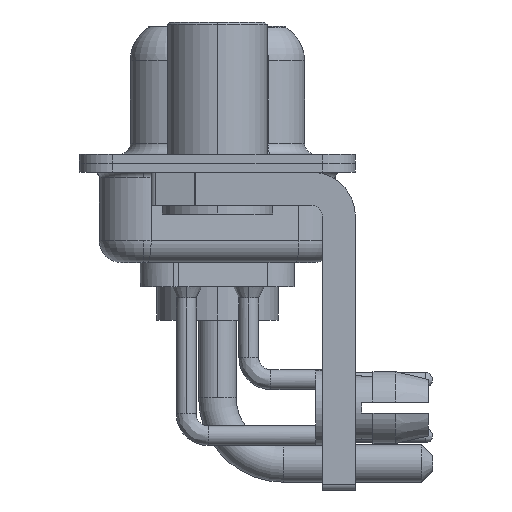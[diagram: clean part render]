
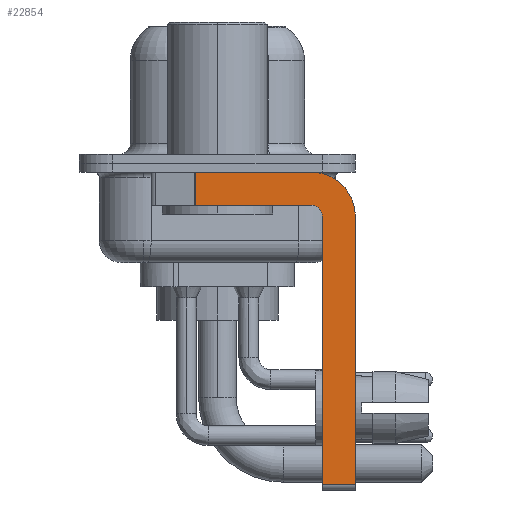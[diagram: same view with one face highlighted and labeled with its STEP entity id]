
A CAD part, left-side view. The second image highlights one B-rep face of the part: STEP entity #22854.
In plain terms, the highlighted planar face has unit normal (-1, 0, 0).
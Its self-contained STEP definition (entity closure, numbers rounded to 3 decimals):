
#73 = CARTESIAN_POINT ( 'NONE',  ( -2.9, -6.25, -2.4 ) ) ;
#445 = LINE ( 'NONE', #2052, #7590 ) ;
#1185 = EDGE_CURVE ( 'NONE', #9826, #1802, #11630, .T. ) ;
#1212 = VERTEX_POINT ( 'NONE', #22719 ) ;
#1387 = DIRECTION ( 'NONE',  ( -1., 0., 0. ) ) ;
#1400 = VECTOR ( 'NONE', #11012, 1000. ) ;
#1431 = EDGE_CURVE ( 'NONE', #19830, #9826, #2947, .T. ) ;
#1802 = VERTEX_POINT ( 'NONE', #73 ) ;
#1924 = ORIENTED_EDGE ( 'NONE', *, *, #15129, .F. ) ;
#2052 = CARTESIAN_POINT ( 'NONE',  ( -2.9, 0.978, -1.9 ) ) ;
#2073 = VERTEX_POINT ( 'NONE', #3316 ) ;
#2643 = EDGE_CURVE ( 'NONE', #7183, #2073, #3138, .T. ) ;
#2680 = PLANE ( 'NONE',  #18071 ) ;
#2716 = ORIENTED_EDGE ( 'NONE', *, *, #20235, .T. ) ;
#2947 = LINE ( 'NONE', #17182, #18067 ) ;
#3077 = CARTESIAN_POINT ( 'NONE',  ( -2.9, -4.25, -1.9 ) ) ;
#3138 = LINE ( 'NONE', #22945, #21038 ) ;
#3316 = CARTESIAN_POINT ( 'NONE',  ( -2.9, -6.25, -14.55 ) ) ;
#4384 = VERTEX_POINT ( 'NONE', #6140 ) ;
#4430 = CARTESIAN_POINT ( 'NONE',  ( -2.9, -4.25, -2.4 ) ) ;
#5725 = DIRECTION ( 'NONE',  ( 0., 0., 1. ) ) ;
#6140 = CARTESIAN_POINT ( 'NONE',  ( -2.9, -4.75, -2.4 ) ) ;
#6662 = CARTESIAN_POINT ( 'NONE',  ( -2.9, -6.25, -2.4 ) ) ;
#6886 = FACE_OUTER_BOUND ( 'NONE', #17686, .T. ) ;
#7026 = DIRECTION ( 'NONE',  ( 0., 0., 1. ) ) ;
#7183 = VERTEX_POINT ( 'NONE', #24680 ) ;
#7384 = CARTESIAN_POINT ( 'NONE',  ( -2.9, 0.978, -0.4 ) ) ;
#7590 = VECTOR ( 'NONE', #20750, 1000. ) ;
#8251 = CARTESIAN_POINT ( 'NONE',  ( -2.9, -4.25, -2.4 ) ) ;
#8667 = DIRECTION ( 'NONE',  ( 1., 0., 0. ) ) ;
#9330 = VECTOR ( 'NONE', #7026, 1000. ) ;
#9657 = ORIENTED_EDGE ( 'NONE', *, *, #1431, .F. ) ;
#9826 = VERTEX_POINT ( 'NONE', #16752 ) ;
#11012 = DIRECTION ( 'NONE',  ( 0., 0., -1. ) ) ;
#11309 = EDGE_CURVE ( 'NONE', #7183, #4384, #13257, .T. ) ;
#11630 = CIRCLE ( 'NONE', #26774, 2. ) ;
#12279 = DIRECTION ( 'NONE',  ( 1., 0., 0. ) ) ;
#12553 = AXIS2_PLACEMENT_3D ( 'NONE', #21988, #1387, #5725 ) ;
#12902 = LINE ( 'NONE', #6662, #1400 ) ;
#12908 = ORIENTED_EDGE ( 'NONE', *, *, #11309, .F. ) ;
#13257 = LINE ( 'NONE', #25590, #9330 ) ;
#13276 = EDGE_CURVE ( 'NONE', #4384, #1212, #22514, .T. ) ;
#15129 = EDGE_CURVE ( 'NONE', #1802, #2073, #12902, .T. ) ;
#16752 = CARTESIAN_POINT ( 'NONE',  ( -2.9, -4.25, -0.4 ) ) ;
#16754 = ORIENTED_EDGE ( 'NONE', *, *, #22962, .F. ) ;
#17182 = CARTESIAN_POINT ( 'NONE',  ( -2.9, 3., -0.4 ) ) ;
#17524 = ORIENTED_EDGE ( 'NONE', *, *, #1185, .F. ) ;
#17686 = EDGE_LOOP ( 'NONE', ( #9657, #2716, #16754, #24186, #12908, #23827, #1924, #17524 ) ) ;
#18067 = VECTOR ( 'NONE', #25715, 1000. ) ;
#18071 = AXIS2_PLACEMENT_3D ( 'NONE', #4430, #8667, #25042 ) ;
#18554 = VERTEX_POINT ( 'NONE', #19426 ) ;
#19426 = CARTESIAN_POINT ( 'NONE',  ( -2.9, 0.978, -1.9 ) ) ;
#19830 = VERTEX_POINT ( 'NONE', #7384 ) ;
#20235 = EDGE_CURVE ( 'NONE', #19830, #18554, #445, .T. ) ;
#20750 = DIRECTION ( 'NONE',  ( 0., 0., -1. ) ) ;
#21038 = VECTOR ( 'NONE', #25266, 1000. ) ;
#21094 = VECTOR ( 'NONE', #22033, 1000. ) ;
#21988 = CARTESIAN_POINT ( 'NONE',  ( -2.9, -4.25, -2.4 ) ) ;
#22033 = DIRECTION ( 'NONE',  ( 0., 1., 0. ) ) ;
#22463 = DIRECTION ( 'NONE',  ( 0., 0., -1. ) ) ;
#22514 = CIRCLE ( 'NONE', #12553, 0.5 ) ;
#22719 = CARTESIAN_POINT ( 'NONE',  ( -2.9, -4.25, -1.9 ) ) ;
#22854 = ADVANCED_FACE ( 'NONE', ( #6886 ), #2680, .F. ) ;
#22945 = CARTESIAN_POINT ( 'NONE',  ( -2.9, -4.25, -14.55 ) ) ;
#22962 = EDGE_CURVE ( 'NONE', #1212, #18554, #26237, .T. ) ;
#23827 = ORIENTED_EDGE ( 'NONE', *, *, #2643, .T. ) ;
#24186 = ORIENTED_EDGE ( 'NONE', *, *, #13276, .F. ) ;
#24680 = CARTESIAN_POINT ( 'NONE',  ( -2.9, -4.75, -14.55 ) ) ;
#25042 = DIRECTION ( 'NONE',  ( 0., 0., -1. ) ) ;
#25266 = DIRECTION ( 'NONE',  ( 0., -1., 0. ) ) ;
#25590 = CARTESIAN_POINT ( 'NONE',  ( -2.9, -4.75, -14.8 ) ) ;
#25715 = DIRECTION ( 'NONE',  ( 0., -1., 0. ) ) ;
#26237 = LINE ( 'NONE', #3077, #21094 ) ;
#26774 = AXIS2_PLACEMENT_3D ( 'NONE', #8251, #12279, #22463 ) ;
